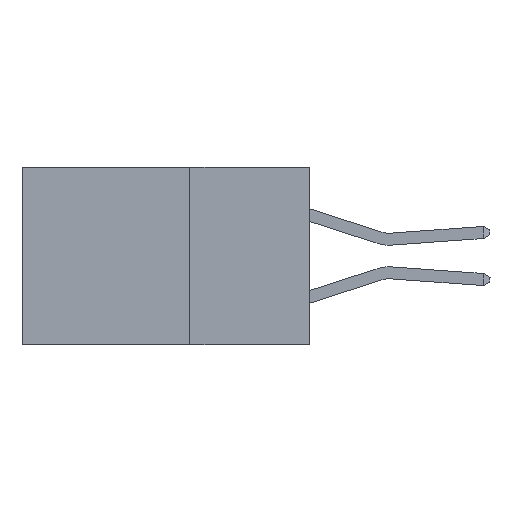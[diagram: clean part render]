
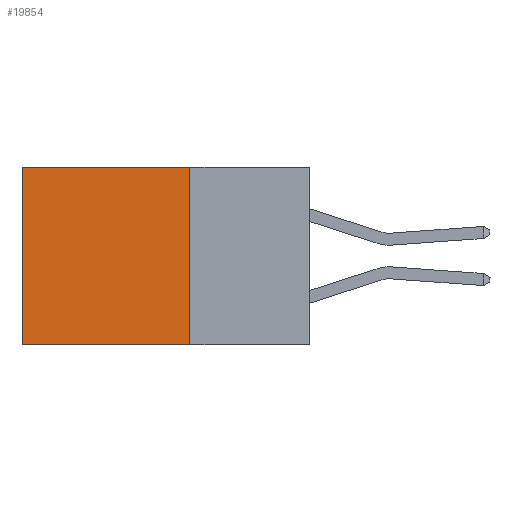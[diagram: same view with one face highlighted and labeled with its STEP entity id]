
A CAD part, left-side view. The second image highlights one B-rep face of the part: STEP entity #19854.
In plain terms, the highlighted planar face has unit normal (-1, 0, 0).
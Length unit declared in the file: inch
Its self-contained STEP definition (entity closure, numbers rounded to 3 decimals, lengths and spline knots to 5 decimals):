
#313 = VERTEX_POINT ( 'NONE', #533 ) ;
#533 = CARTESIAN_POINT ( 'NONE',  ( 0.2615, 0.25, -0.37 ) ) ;
#1069 = LINE ( 'NONE', #7614, #10611 ) ;
#1095 = LINE ( 'NONE', #17803, #15683 ) ;
#5026 = DIRECTION ( 'NONE',  ( 1., 0., 0. ) ) ;
#5869 = EDGE_CURVE ( 'NONE', #16991, #313, #1095, .T. ) ;
#6377 = EDGE_CURVE ( 'NONE', #313, #21989, #1069, .T. ) ;
#6866 = CARTESIAN_POINT ( 'NONE',  ( 0.2615, 0.25, -0.37 ) ) ;
#7015 = EDGE_LOOP ( 'NONE', ( #8716, #9504, #18593, #23080 ) ) ;
#7504 = DIRECTION ( 'NONE',  ( 0., 1., 0. ) ) ;
#7508 = CARTESIAN_POINT ( 'NONE',  ( 0.2615, 0.6, -0.37 ) ) ;
#7614 = CARTESIAN_POINT ( 'NONE',  ( 0.2615, 0.25, -0.37 ) ) ;
#7910 = CARTESIAN_POINT ( 'NONE',  ( 0.2615, 0.6, 0. ) ) ;
#8716 = ORIENTED_EDGE ( 'NONE', *, *, #20672, .T. ) ;
#9104 = DIRECTION ( 'NONE',  ( 0., 1., 0. ) ) ;
#9504 = ORIENTED_EDGE ( 'NONE', *, *, #6377, .F. ) ;
#9969 = VERTEX_POINT ( 'NONE', #7910 ) ;
#10611 = VECTOR ( 'NONE', #7504, 39.37008 ) ;
#12599 = EDGE_CURVE ( 'NONE', #16991, #9969, #20247, .T. ) ;
#13655 = AXIS2_PLACEMENT_3D ( 'NONE', #6866, #5026, #18380 ) ;
#14014 = CARTESIAN_POINT ( 'NONE',  ( 0.2615, 0.25, 0. ) ) ;
#15683 = VECTOR ( 'NONE', #17246, 39.37008 ) ;
#16487 = PLANE ( 'NONE',  #13655 ) ;
#16991 = VERTEX_POINT ( 'NONE', #14014 ) ;
#17152 = CARTESIAN_POINT ( 'NONE',  ( 0.2615, 0.6, -0.37 ) ) ;
#17246 = DIRECTION ( 'NONE',  ( 0., 0., -1. ) ) ;
#17426 = DIRECTION ( 'NONE',  ( 0., 0., -1. ) ) ;
#17803 = CARTESIAN_POINT ( 'NONE',  ( 0.2615, 0.25, -0.37 ) ) ;
#18380 = DIRECTION ( 'NONE',  ( 0., 0., -1. ) ) ;
#18593 = ORIENTED_EDGE ( 'NONE', *, *, #5869, .F. ) ;
#19652 = FACE_OUTER_BOUND ( 'NONE', #7015, .T. ) ;
#19854 = ADVANCED_FACE ( 'NONE', ( #19652 ), #16487, .F. ) ;
#20247 = LINE ( 'NONE', #22396, #20875 ) ;
#20672 = EDGE_CURVE ( 'NONE', #9969, #21989, #23455, .T. ) ;
#20875 = VECTOR ( 'NONE', #9104, 39.37008 ) ;
#21989 = VERTEX_POINT ( 'NONE', #17152 ) ;
#22396 = CARTESIAN_POINT ( 'NONE',  ( 0.2615, 0.25, 0. ) ) ;
#22894 = VECTOR ( 'NONE', #17426, 39.37008 ) ;
#23080 = ORIENTED_EDGE ( 'NONE', *, *, #12599, .T. ) ;
#23455 = LINE ( 'NONE', #7508, #22894 ) ;
